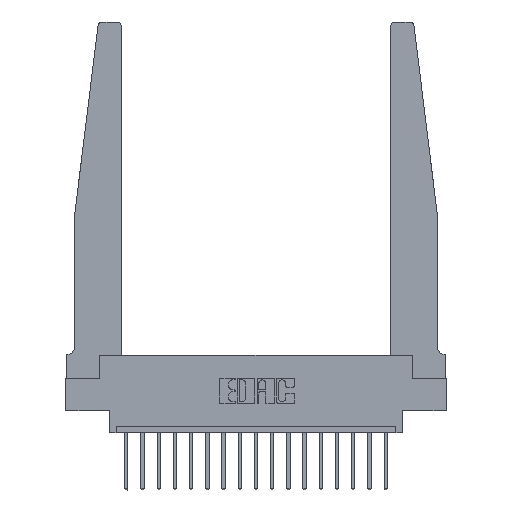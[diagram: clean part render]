
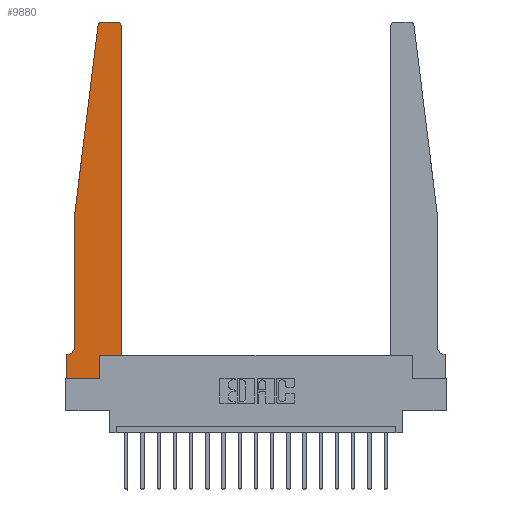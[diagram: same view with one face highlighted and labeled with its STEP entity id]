
A CAD part, top view. The second image highlights one B-rep face of the part: STEP entity #9880.
In plain terms, the highlighted planar face has unit normal (0, 0, 1).
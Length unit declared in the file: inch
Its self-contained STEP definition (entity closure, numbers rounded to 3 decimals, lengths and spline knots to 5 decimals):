
#133 = CARTESIAN_POINT ( 'NONE',  ( 0.2605, 0.18, 0.37 ) ) ;
#435 = CARTESIAN_POINT ( 'NONE',  ( 0.24675, 2.72367, 0.37 ) ) ;
#761 = ORIENTED_EDGE ( 'NONE', *, *, #13184, .T. ) ;
#813 = DIRECTION ( 'NONE',  ( 1., 0., 0. ) ) ;
#863 = EDGE_CURVE ( 'NONE', #9651, #18395, #4839, .T. ) ;
#1083 = EDGE_CURVE ( 'NONE', #13328, #7165, #7320, .T. ) ;
#1241 = ORIENTED_EDGE ( 'NONE', *, *, #5681, .T. ) ;
#1300 = EDGE_CURVE ( 'NONE', #5746, #2429, #10057, .T. ) ;
#1309 = DIRECTION ( 'NONE',  ( 0., -1., 0. ) ) ;
#1637 = ORIENTED_EDGE ( 'NONE', *, *, #5628, .T. ) ;
#1754 = CARTESIAN_POINT ( 'NONE',  ( 0., 0.1875, 0.37 ) ) ;
#2001 = DIRECTION ( 'NONE',  ( 0., 0., 1. ) ) ;
#2019 = CARTESIAN_POINT ( 'NONE',  ( 0.425, 0.18, 0.37 ) ) ;
#2055 = EDGE_CURVE ( 'NONE', #3634, #5746, #5473, .T. ) ;
#2057 = ORIENTED_EDGE ( 'NONE', *, *, #4560, .T. ) ;
#2353 = CARTESIAN_POINT ( 'NONE',  ( 0.27653, 2.75, 0.37 ) ) ;
#2429 = VERTEX_POINT ( 'NONE', #1754 ) ;
#2481 = AXIS2_PLACEMENT_3D ( 'NONE', #10225, #7415, #8688 ) ;
#3320 = EDGE_CURVE ( 'NONE', #7165, #16771, #16590, .T. ) ;
#3431 = CIRCLE ( 'NONE', #18503, 0.03 ) ;
#3634 = VERTEX_POINT ( 'NONE', #7861 ) ;
#3645 = CARTESIAN_POINT ( 'NONE',  ( 0., 0.1875, 0.37 ) ) ;
#3708 = VECTOR ( 'NONE', #15684, 39.37008 ) ;
#3735 = ORIENTED_EDGE ( 'NONE', *, *, #16835, .T. ) ;
#4560 = EDGE_CURVE ( 'NONE', #18231, #11114, #4700, .T. ) ;
#4700 = LINE ( 'NONE', #13400, #5134 ) ;
#4747 = ORIENTED_EDGE ( 'NONE', *, *, #863, .T. ) ;
#4827 = AXIS2_PLACEMENT_3D ( 'NONE', #3645, #6560, #813 ) ;
#4839 = LINE ( 'NONE', #2019, #15557 ) ;
#4910 = ORIENTED_EDGE ( 'NONE', *, *, #9477, .T. ) ;
#4986 = DIRECTION ( 'NONE',  ( 0., 1., 0. ) ) ;
#5134 = VECTOR ( 'NONE', #7405, 39.37008 ) ;
#5473 = CIRCLE ( 'NONE', #2481, 0.05 ) ;
#5628 = EDGE_CURVE ( 'NONE', #7470, #18231, #18046, .T. ) ;
#5681 = EDGE_CURVE ( 'NONE', #15538, #7470, #16055, .T. ) ;
#5746 = VERTEX_POINT ( 'NONE', #6977 ) ;
#6020 = LINE ( 'NONE', #11319, #14229 ) ;
#6398 = CARTESIAN_POINT ( 'NONE',  ( 0.395, 2.75, 0.37 ) ) ;
#6560 = DIRECTION ( 'NONE',  ( 0., 0., 1. ) ) ;
#6646 = EDGE_LOOP ( 'NONE', ( #1241, #1637, #2057, #4910, #7841, #16856, #10956, #8363, #13754, #3735, #4747, #761 ) ) ;
#6852 = CARTESIAN_POINT ( 'NONE',  ( 0.25, 2.75, 0.37 ) ) ;
#6977 = CARTESIAN_POINT ( 'NONE',  ( 0.015, 0.1875, 0.37 ) ) ;
#7158 = FACE_OUTER_BOUND ( 'NONE', #6646, .T. ) ;
#7165 = VERTEX_POINT ( 'NONE', #13940 ) ;
#7174 = VECTOR ( 'NONE', #1309, 39.37008 ) ;
#7228 = DIRECTION ( 'NONE',  ( 0., 1., 0. ) ) ;
#7320 = LINE ( 'NONE', #17983, #11450 ) ;
#7405 = DIRECTION ( 'NONE',  ( -0.122, -0.992, 0. ) ) ;
#7415 = DIRECTION ( 'NONE',  ( 0., 0., -1. ) ) ;
#7470 = VERTEX_POINT ( 'NONE', #2353 ) ;
#7819 = CARTESIAN_POINT ( 'NONE',  ( 0.065, 0.1875, 0.37 ) ) ;
#7841 = ORIENTED_EDGE ( 'NONE', *, *, #2055, .T. ) ;
#7861 = CARTESIAN_POINT ( 'NONE',  ( 0.065, 0.2375, 0.37 ) ) ;
#8095 = VECTOR ( 'NONE', #11743, 39.37008 ) ;
#8363 = ORIENTED_EDGE ( 'NONE', *, *, #1083, .T. ) ;
#8680 = CARTESIAN_POINT ( 'NONE',  ( 0.425, 0.18, 0.37 ) ) ;
#8688 = DIRECTION ( 'NONE',  ( -1., 0., 0. ) ) ;
#8818 = VECTOR ( 'NONE', #7228, 39.37008 ) ;
#9214 = DIRECTION ( 'NONE',  ( -1., 0., 0. ) ) ;
#9417 = PLANE ( 'NONE',  #4827 ) ;
#9468 = LINE ( 'NONE', #8680, #8095 ) ;
#9477 = EDGE_CURVE ( 'NONE', #11114, #3634, #9929, .T. ) ;
#9651 = VERTEX_POINT ( 'NONE', #16010 ) ;
#9880 = ADVANCED_FACE ( 'NONE', ( #7158 ), #9417, .T. ) ;
#9929 = LINE ( 'NONE', #15767, #7174 ) ;
#10057 = LINE ( 'NONE', #7819, #12808 ) ;
#10225 = CARTESIAN_POINT ( 'NONE',  ( 0.015, 0.2375, 0.37 ) ) ;
#10690 = CARTESIAN_POINT ( 'NONE',  ( 0.395, 2.72, 0.37 ) ) ;
#10956 = ORIENTED_EDGE ( 'NONE', *, *, #17934, .T. ) ;
#11054 = DIRECTION ( 'NONE',  ( 1., 0., 0. ) ) ;
#11114 = VERTEX_POINT ( 'NONE', #16110 ) ;
#11319 = CARTESIAN_POINT ( 'NONE',  ( 0., 0., 0.37 ) ) ;
#11450 = VECTOR ( 'NONE', #11054, 39.37008 ) ;
#11743 = DIRECTION ( 'NONE',  ( 1., 0., 0. ) ) ;
#12144 = DIRECTION ( 'NONE',  ( 1., 0., 0. ) ) ;
#12808 = VECTOR ( 'NONE', #9214, 39.37008 ) ;
#13184 = EDGE_CURVE ( 'NONE', #18395, #15538, #3431, .T. ) ;
#13328 = VERTEX_POINT ( 'NONE', #14972 ) ;
#13400 = CARTESIAN_POINT ( 'NONE',  ( 0.065, 1.25, 0.37 ) ) ;
#13754 = ORIENTED_EDGE ( 'NONE', *, *, #3320, .T. ) ;
#13921 = DIRECTION ( 'NONE',  ( 0., -1., 0. ) ) ;
#13940 = CARTESIAN_POINT ( 'NONE',  ( 0.2605, 0., 0.37 ) ) ;
#14229 = VECTOR ( 'NONE', #13921, 39.37008 ) ;
#14951 = CARTESIAN_POINT ( 'NONE',  ( 0.27653, 2.72, 0.37 ) ) ;
#14972 = CARTESIAN_POINT ( 'NONE',  ( 0., 0., 0.37 ) ) ;
#15538 = VERTEX_POINT ( 'NONE', #6398 ) ;
#15557 = VECTOR ( 'NONE', #4986, 39.37008 ) ;
#15662 = CARTESIAN_POINT ( 'NONE',  ( 0.2605, 0.18, 0.37 ) ) ;
#15684 = DIRECTION ( 'NONE',  ( -1., 0., 0. ) ) ;
#15767 = CARTESIAN_POINT ( 'NONE',  ( 0.065, 1.25, 0.37 ) ) ;
#15800 = AXIS2_PLACEMENT_3D ( 'NONE', #14951, #16512, #17919 ) ;
#16010 = CARTESIAN_POINT ( 'NONE',  ( 0.425, 0.18, 0.37 ) ) ;
#16055 = LINE ( 'NONE', #6852, #3708 ) ;
#16110 = CARTESIAN_POINT ( 'NONE',  ( 0.065, 1.25, 0.37 ) ) ;
#16512 = DIRECTION ( 'NONE',  ( 0., 0., 1. ) ) ;
#16590 = LINE ( 'NONE', #133, #8818 ) ;
#16771 = VERTEX_POINT ( 'NONE', #15662 ) ;
#16835 = EDGE_CURVE ( 'NONE', #16771, #9651, #9468, .T. ) ;
#16856 = ORIENTED_EDGE ( 'NONE', *, *, #1300, .T. ) ;
#17919 = DIRECTION ( 'NONE',  ( 1., 0., 0. ) ) ;
#17934 = EDGE_CURVE ( 'NONE', #2429, #13328, #6020, .T. ) ;
#17983 = CARTESIAN_POINT ( 'NONE',  ( 0., 0., 0.37 ) ) ;
#18046 = CIRCLE ( 'NONE', #15800, 0.03 ) ;
#18231 = VERTEX_POINT ( 'NONE', #435 ) ;
#18328 = CARTESIAN_POINT ( 'NONE',  ( 0.425, 2.72, 0.37 ) ) ;
#18395 = VERTEX_POINT ( 'NONE', #18328 ) ;
#18503 = AXIS2_PLACEMENT_3D ( 'NONE', #10690, #2001, #12144 ) ;
